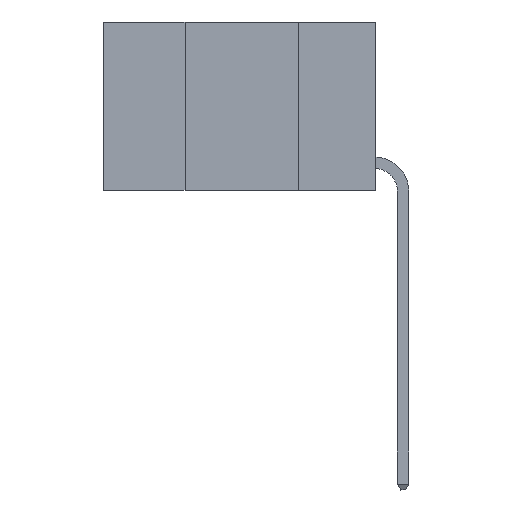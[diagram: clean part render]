
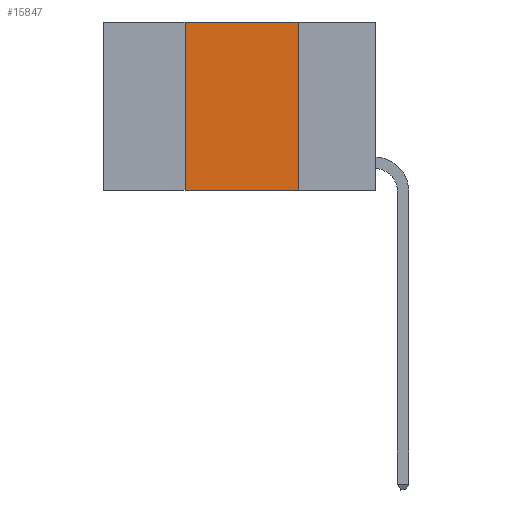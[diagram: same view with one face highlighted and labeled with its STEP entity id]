
A CAD part, left-side view. The second image highlights one B-rep face of the part: STEP entity #15847.
In plain terms, the highlighted planar face has unit normal (-1, 0, 0).
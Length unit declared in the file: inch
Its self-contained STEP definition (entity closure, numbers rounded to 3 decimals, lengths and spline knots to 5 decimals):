
#30 = CARTESIAN_POINT ( 'NONE',  ( 0., 0.6, -0.37 ) ) ;
#1200 = VERTEX_POINT ( 'NONE', #10079 ) ;
#1631 = DIRECTION ( 'NONE',  ( 0., -1., 0. ) ) ;
#1939 = EDGE_CURVE ( 'NONE', #16468, #18841, #11317, .T. ) ;
#2172 = LINE ( 'NONE', #30, #10125 ) ;
#3806 = CARTESIAN_POINT ( 'NONE',  ( 0., 0.42, 0. ) ) ;
#4187 = VECTOR ( 'NONE', #12556, 39.37008 ) ;
#4460 = EDGE_CURVE ( 'NONE', #11290, #16468, #10225, .T. ) ;
#5592 = PLANE ( 'NONE',  #16492 ) ;
#5905 = EDGE_CURVE ( 'NONE', #18841, #1200, #13763, .T. ) ;
#6020 = EDGE_CURVE ( 'NONE', #11290, #1200, #2172, .T. ) ;
#6446 = CARTESIAN_POINT ( 'NONE',  ( 0., 0.42, -0.37 ) ) ;
#6623 = VECTOR ( 'NONE', #15665, 39.37008 ) ;
#7188 = DIRECTION ( 'NONE',  ( 1., 0., 0. ) ) ;
#8584 = ORIENTED_EDGE ( 'NONE', *, *, #1939, .F. ) ;
#8609 = ORIENTED_EDGE ( 'NONE', *, *, #6020, .T. ) ;
#9736 = VECTOR ( 'NONE', #15081, 39.37008 ) ;
#10079 = CARTESIAN_POINT ( 'NONE',  ( 0., 0.17, -0.37 ) ) ;
#10125 = VECTOR ( 'NONE', #1631, 39.37008 ) ;
#10225 = LINE ( 'NONE', #3806, #9736 ) ;
#10561 = EDGE_LOOP ( 'NONE', ( #12385, #8584, #18350, #8609 ) ) ;
#10852 = CARTESIAN_POINT ( 'NONE',  ( 0., 0.17, 0. ) ) ;
#11290 = VERTEX_POINT ( 'NONE', #6446 ) ;
#11317 = LINE ( 'NONE', #15802, #6623 ) ;
#11524 = FACE_OUTER_BOUND ( 'NONE', #10561, .T. ) ;
#12385 = ORIENTED_EDGE ( 'NONE', *, *, #5905, .F. ) ;
#12556 = DIRECTION ( 'NONE',  ( 0., 0., -1. ) ) ;
#13763 = LINE ( 'NONE', #10852, #4187 ) ;
#15073 = CARTESIAN_POINT ( 'NONE',  ( 0., 0.17, 0. ) ) ;
#15081 = DIRECTION ( 'NONE',  ( 0., 0., 1. ) ) ;
#15665 = DIRECTION ( 'NONE',  ( 0., -1., 0. ) ) ;
#15802 = CARTESIAN_POINT ( 'NONE',  ( 0., 0.6, 0. ) ) ;
#15847 = ADVANCED_FACE ( 'NONE', ( #11524 ), #5592, .F. ) ;
#16468 = VERTEX_POINT ( 'NONE', #19418 ) ;
#16492 = AXIS2_PLACEMENT_3D ( 'NONE', #16815, #7188, #18354 ) ;
#16815 = CARTESIAN_POINT ( 'NONE',  ( 0., 0.6, 0. ) ) ;
#18350 = ORIENTED_EDGE ( 'NONE', *, *, #4460, .F. ) ;
#18354 = DIRECTION ( 'NONE',  ( 0., 0., -1. ) ) ;
#18841 = VERTEX_POINT ( 'NONE', #15073 ) ;
#19418 = CARTESIAN_POINT ( 'NONE',  ( 0., 0.42, 0. ) ) ;
